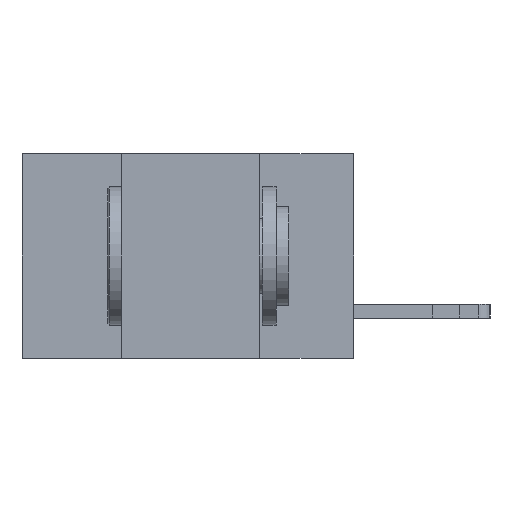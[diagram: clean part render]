
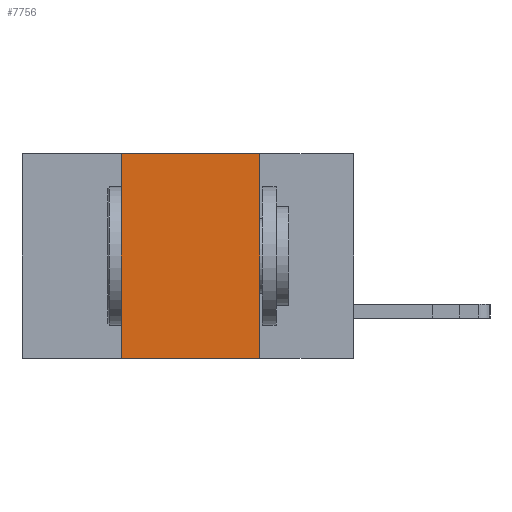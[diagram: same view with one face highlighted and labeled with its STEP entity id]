
A CAD part, left-side view. The second image highlights one B-rep face of the part: STEP entity #7756.
In plain terms, the highlighted planar face has unit normal (-1, 0, 0).
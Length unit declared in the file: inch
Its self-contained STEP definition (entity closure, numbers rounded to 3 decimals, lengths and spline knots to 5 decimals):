
#270 = DIRECTION ( 'NONE',  ( 0., -1., 0. ) ) ;
#668 = AXIS2_PLACEMENT_3D ( 'NONE', #15309, #6105, #12652 ) ;
#669 = CARTESIAN_POINT ( 'NONE',  ( 0., 0.17, -0.37 ) ) ;
#1128 = VECTOR ( 'NONE', #270, 39.37008 ) ;
#1761 = DIRECTION ( 'NONE',  ( 0., -1., 0. ) ) ;
#2729 = EDGE_CURVE ( 'NONE', #12321, #15943, #8332, .T. ) ;
#3134 = ORIENTED_EDGE ( 'NONE', *, *, #10777, .F. ) ;
#3368 = VERTEX_POINT ( 'NONE', #3712 ) ;
#3404 = VECTOR ( 'NONE', #14790, 39.37008 ) ;
#3676 = FACE_OUTER_BOUND ( 'NONE', #3955, .T. ) ;
#3712 = CARTESIAN_POINT ( 'NONE',  ( 0., 0.17, 0. ) ) ;
#3955 = EDGE_LOOP ( 'NONE', ( #9682, #3134, #12115, #10227 ) ) ;
#4250 = LINE ( 'NONE', #9488, #7343 ) ;
#4384 = LINE ( 'NONE', #14546, #3404 ) ;
#4611 = VERTEX_POINT ( 'NONE', #4775 ) ;
#4775 = CARTESIAN_POINT ( 'NONE',  ( 0., 0.42, 0. ) ) ;
#4901 = EDGE_CURVE ( 'NONE', #12321, #4611, #4250, .T. ) ;
#5561 = VECTOR ( 'NONE', #1761, 39.37008 ) ;
#5752 = CARTESIAN_POINT ( 'NONE',  ( 0., 0.6, -0.37 ) ) ;
#6105 = DIRECTION ( 'NONE',  ( 1., 0., 0. ) ) ;
#7343 = VECTOR ( 'NONE', #8212, 39.37008 ) ;
#7756 = ADVANCED_FACE ( 'NONE', ( #3676 ), #10041, .F. ) ;
#8212 = DIRECTION ( 'NONE',  ( 0., 0., 1. ) ) ;
#8332 = LINE ( 'NONE', #5752, #1128 ) ;
#9488 = CARTESIAN_POINT ( 'NONE',  ( 0., 0.42, 0. ) ) ;
#9682 = ORIENTED_EDGE ( 'NONE', *, *, #14239, .F. ) ;
#9831 = CARTESIAN_POINT ( 'NONE',  ( 0., 0.42, -0.37 ) ) ;
#10041 = PLANE ( 'NONE',  #668 ) ;
#10227 = ORIENTED_EDGE ( 'NONE', *, *, #2729, .T. ) ;
#10777 = EDGE_CURVE ( 'NONE', #4611, #3368, #14580, .T. ) ;
#12115 = ORIENTED_EDGE ( 'NONE', *, *, #4901, .F. ) ;
#12321 = VERTEX_POINT ( 'NONE', #9831 ) ;
#12652 = DIRECTION ( 'NONE',  ( 0., 0., -1. ) ) ;
#14239 = EDGE_CURVE ( 'NONE', #3368, #15943, #4384, .T. ) ;
#14546 = CARTESIAN_POINT ( 'NONE',  ( 0., 0.17, 0. ) ) ;
#14580 = LINE ( 'NONE', #14746, #5561 ) ;
#14746 = CARTESIAN_POINT ( 'NONE',  ( 0., 0.6, 0. ) ) ;
#14790 = DIRECTION ( 'NONE',  ( 0., 0., -1. ) ) ;
#15309 = CARTESIAN_POINT ( 'NONE',  ( 0., 0.6, 0. ) ) ;
#15943 = VERTEX_POINT ( 'NONE', #669 ) ;
